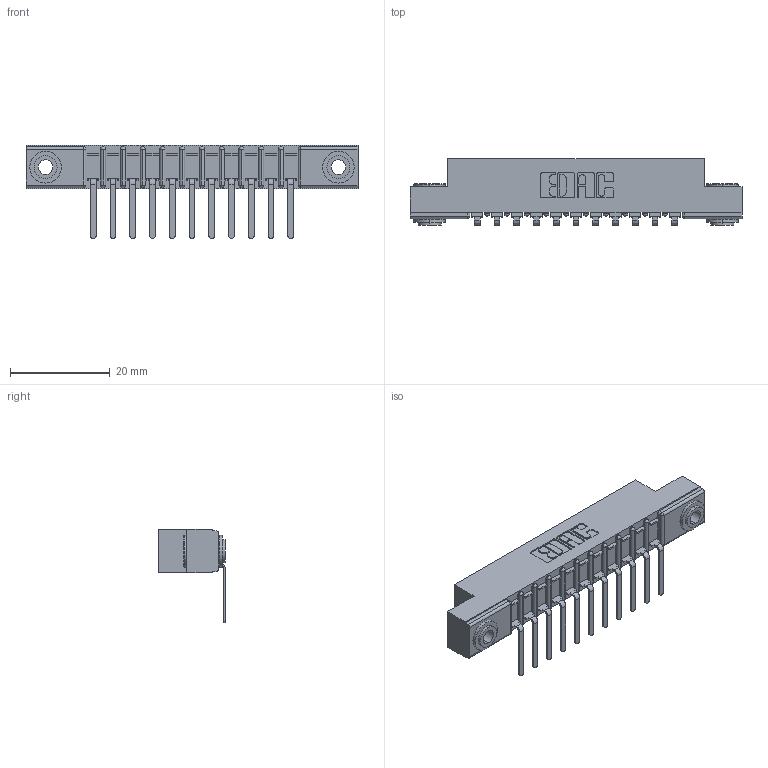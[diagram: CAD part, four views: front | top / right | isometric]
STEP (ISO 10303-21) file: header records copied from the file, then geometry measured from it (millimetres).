
FILE_DESCRIPTION (( 'STEP AP203' ), '1' );
FILE_NAME ('307-011-457-103.STEP', '2020-09-25T10:53:18', ( '' ), ( '' ), 'SwSTEP 2.0', 'SolidWorks 2020', '' );
FILE_SCHEMA (( 'CONFIG_CONTROL_DESIGN' ));
Length unit declared in the file: inch
Products named in the file (4): 345-250-002_345-250-002-102; 307-011-457-103; 307 Part_.156 Dia Mounting Holes; 307-290-002_557
Assembly tree (14 placements, depth 2):
  307-011-457-103
    307 Part_.156 Dia Mounting Holes
    307-290-002_557  x11
    345-250-002_345-250-002-102  x2
Bounding box: 66.6 x 13.36 x 18.67 mm (x, y, z)
Volume: 4422 mm3; surface area: 7856.5 mm2
Topology: 14 solids, 14 shells, 1040 faces, 3119 edges, 2042 vertices
Faces by surface type: plane 611, cylinder 397, sphere 24, cone 8
Entity records: 15171 total; most frequent: CARTESIAN_POINT 2533, ORIENTED_EDGE 2514, DIRECTION 2491, EDGE_CURVE 1257, LINE 939, VECTOR 939, VERTEX_POINT 818, AXIS2_PLACEMENT_3D 776
